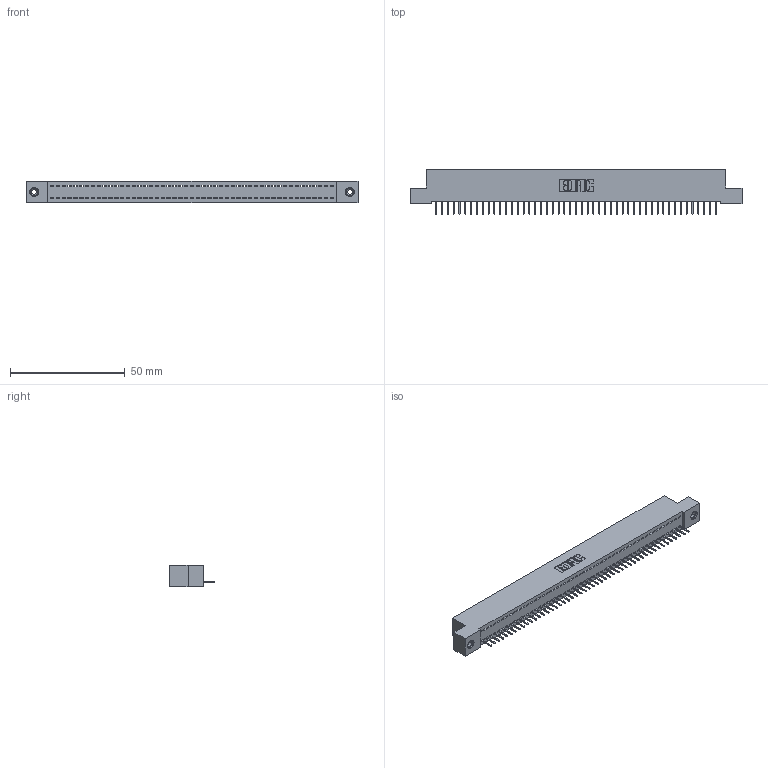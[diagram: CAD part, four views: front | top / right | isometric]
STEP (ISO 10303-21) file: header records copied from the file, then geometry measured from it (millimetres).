
FILE_DESCRIPTION (( 'STEP AP203' ), '1' );
FILE_NAME ('342-049-524-108.STEP', '2018-08-12T18:53:31', ( '' ), ( '' ), 'SwSTEP 2.0', 'SolidWorks 2016', '' );
FILE_SCHEMA (( 'CONFIG_CONTROL_DESIGN' ));
Length unit declared in the file: inch
Products named in the file (4): 342 Part_TI; 345-292-001_345-293-124; 345-250-001_345-250-003-102; 342-049-524-108
Assembly tree (52 placements, depth 2):
  342-049-524-108
    342 Part_TI
    345-292-001_345-293-124  x49
    345-250-001_345-250-003-102  x2
Bounding box: 144.78 x 19.69 x 9.4 mm (x, y, z)
Volume: 12520.9 mm3; surface area: 17933.6 mm2
Topology: 52 solids, 52 shells, 3208 faces, 9255 edges, 5966 vertices
Faces by surface type: plane 2450, cylinder 742, cone 12, torus 4
Entity records: 30178 total; most frequent: CARTESIAN_POINT 5184, ORIENTED_EDGE 5162, DIRECTION 4393, EDGE_CURVE 2581, LINE 2437, VECTOR 2437, VERTEX_POINT 1712, AXIS2_PLACEMENT_3D 978
